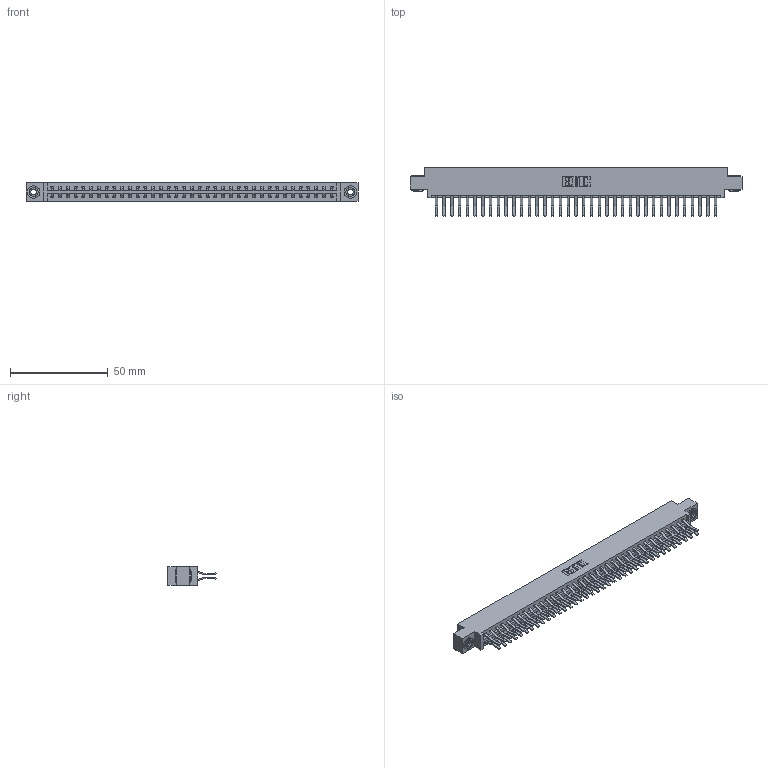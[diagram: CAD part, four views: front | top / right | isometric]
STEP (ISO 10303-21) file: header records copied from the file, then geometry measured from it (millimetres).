
FILE_DESCRIPTION (( 'STEP AP203' ), '1' );
FILE_NAME ('387-074-560-803.STEP', '2018-09-22T20:50:19', ( '' ), ( '' ), 'SwSTEP 2.0', 'SolidWorks 2016', '' );
FILE_SCHEMA (( 'CONFIG_CONTROL_DESIGN' ));
Length unit declared in the file: inch
Products named in the file (4): 337 Part_0.170 Offset - 0.156 Dia-TH; 345-292-001_560 Tail; 345-250-002_345-250-002-102; 387-074-560-803
Assembly tree (77 placements, depth 2):
  387-074-560-803
    337 Part_0.170 Offset - 0.156 Dia-TH
    345-292-001_560 Tail  x74
    345-250-002_345-250-002-102  x2
Bounding box: 169.62 x 24.78 x 9.4 mm (x, y, z)
Volume: 18196.4 mm3; surface area: 22258.6 mm2
Topology: 77 solids, 77 shells, 4300 faces, 12757 edges, 8402 vertices
Faces by surface type: plane 2896, cylinder 1396, cone 8
Entity records: 30204 total; most frequent: CARTESIAN_POINT 5069, ORIENTED_EDGE 4998, DIRECTION 4357, EDGE_CURVE 2499, LINE 2343, VECTOR 2343, VERTEX_POINT 1662, AXIS2_PLACEMENT_3D 1007
